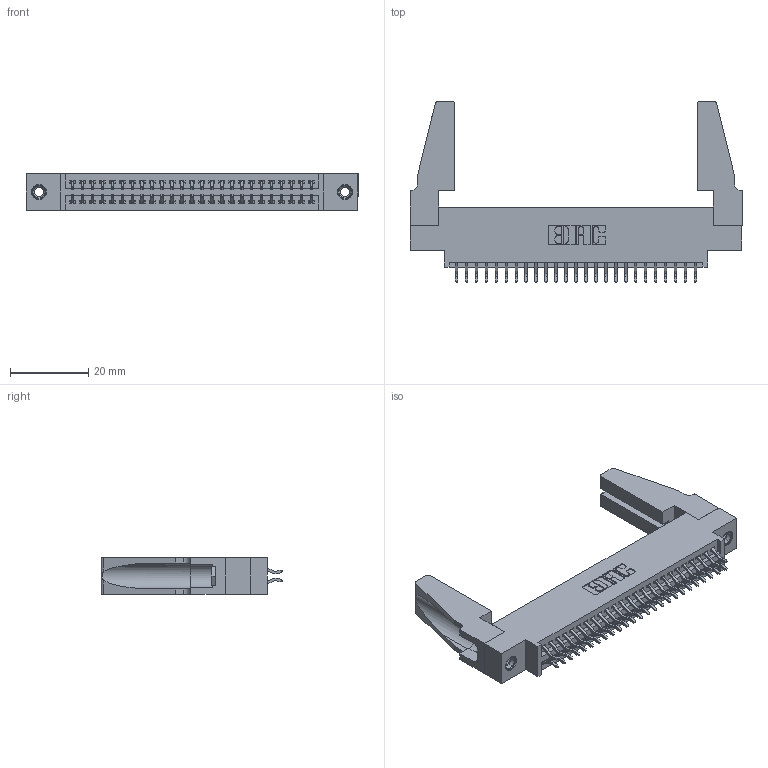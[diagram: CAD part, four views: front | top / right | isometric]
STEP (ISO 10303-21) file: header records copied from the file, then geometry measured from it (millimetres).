
FILE_DESCRIPTION (( 'STEP AP203' ), '1' );
FILE_NAME ('395-050-556-888.STEP', '2019-10-19T14:07:39', ( '' ), ( '' ), 'SwSTEP 2.0', 'SolidWorks 2016', '' );
FILE_SCHEMA (( 'CONFIG_CONTROL_DESIGN' ));
Length unit declared in the file: inch
Products named in the file (5): 345-292-001_556 Tail; 345-250-001_345-250-001-102; 345-220-078_345-220-088; 395-050-556-888; 345 Part_0.170 Offset - 0.156 Dia-TH
Assembly tree (55 placements, depth 2):
  395-050-556-888
    345 Part_0.170 Offset - 0.156 Dia-TH
    345-292-001_556 Tail  x50
    345-250-001_345-250-001-102  x2
    345-220-078_345-220-088  x2
Bounding box: 84.73 x 46.41 x 9.4 mm (x, y, z)
Volume: 11210.5 mm3; surface area: 14655.9 mm2
Topology: 55 solids, 55 shells, 3054 faces, 9017 edges, 5934 vertices
Faces by surface type: plane 2006, cylinder 1032, cone 12, torus 4
Entity records: 24404 total; most frequent: CARTESIAN_POINT 4118, ORIENTED_EDGE 4000, DIRECTION 3644, EDGE_CURVE 2000, VECTOR 1718, LINE 1718, VERTEX_POINT 1326, AXIS2_PLACEMENT_3D 963
